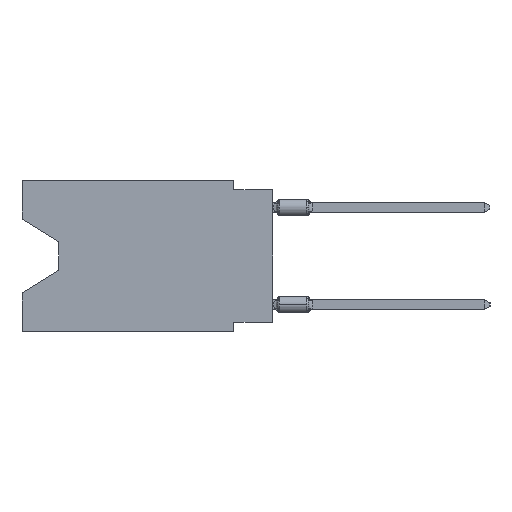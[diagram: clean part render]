
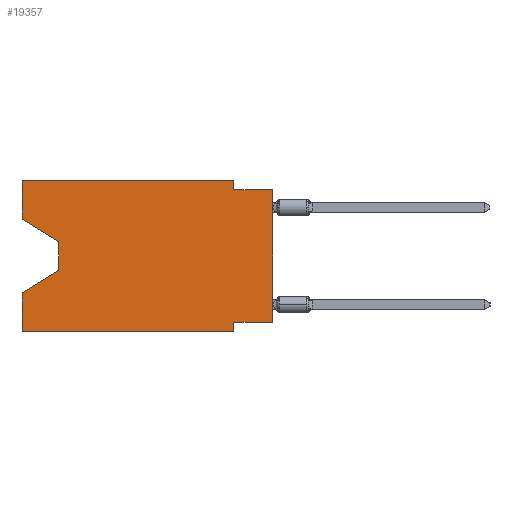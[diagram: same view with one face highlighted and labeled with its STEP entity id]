
A CAD part, left-side view. The second image highlights one B-rep face of the part: STEP entity #19357.
In plain terms, the highlighted planar face has unit normal (-1, 0, 0).
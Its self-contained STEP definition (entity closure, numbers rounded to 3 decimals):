
#1001 = CARTESIAN_POINT ( 'NONE',  ( 0., 0., -9.271 ) ) ;
#1278 = CARTESIAN_POINT ( 'NONE',  ( 0., 16.383, -9.906 ) ) ;
#1820 = CARTESIAN_POINT ( 'NONE',  ( 0., 16.383, 0. ) ) ;
#2032 = VERTEX_POINT ( 'NONE', #52408 ) ;
#2123 = EDGE_CURVE ( 'NONE', #40672, #59513, #11271, .T. ) ;
#3144 = CARTESIAN_POINT ( 'NONE',  ( 0., 2.54, -0.635 ) ) ;
#3154 = DIRECTION ( 'NONE',  ( 0., -0.855, -0.519 ) ) ;
#3254 = LINE ( 'NONE', #39486, #27759 ) ;
#4217 = DIRECTION ( 'NONE',  ( 0., 0., 1. ) ) ;
#4547 = VECTOR ( 'NONE', #3154, 1000. ) ;
#6039 = VECTOR ( 'NONE', #48702, 1000. ) ;
#7146 = LINE ( 'NONE', #20957, #4547 ) ;
#11271 = LINE ( 'NONE', #29998, #6039 ) ;
#11551 = CARTESIAN_POINT ( 'NONE',  ( 0., 13.97, -5.893 ) ) ;
#12085 = VECTOR ( 'NONE', #20526, 1000. ) ;
#12432 = VECTOR ( 'NONE', #40682, 1000. ) ;
#12573 = VECTOR ( 'NONE', #15448, 1000. ) ;
#12969 = EDGE_LOOP ( 'NONE', ( #15234, #33866, #51810, #21047, #34002, #48993, #49906, #43715, #22355, #38930, #28117, #49128 ) ) ;
#13271 = FACE_OUTER_BOUND ( 'NONE', #12969, .T. ) ;
#13844 = VECTOR ( 'NONE', #4217, 1000. ) ;
#14846 = CARTESIAN_POINT ( 'NONE',  ( 0., 2.54, -9.906 ) ) ;
#15234 = ORIENTED_EDGE ( 'NONE', *, *, #43062, .T. ) ;
#15448 = DIRECTION ( 'NONE',  ( 0., 0.855, -0.519 ) ) ;
#16613 = CARTESIAN_POINT ( 'NONE',  ( 0., 13.97, -4.013 ) ) ;
#17149 = CARTESIAN_POINT ( 'NONE',  ( 0., 0., -9.271 ) ) ;
#19357 = ADVANCED_FACE ( 'NONE', ( #13271 ), #56511, .F. ) ;
#19986 = DIRECTION ( 'NONE',  ( 0., -1., 0. ) ) ;
#20526 = DIRECTION ( 'NONE',  ( 0., -1., 0. ) ) ;
#20957 = CARTESIAN_POINT ( 'NONE',  ( 0., 16.383, -2.546 ) ) ;
#21047 = ORIENTED_EDGE ( 'NONE', *, *, #49150, .F. ) ;
#21268 = LINE ( 'NONE', #39997, #27341 ) ;
#22106 = DIRECTION ( 'NONE',  ( 0., 0., -1. ) ) ;
#22355 = ORIENTED_EDGE ( 'NONE', *, *, #46627, .F. ) ;
#23668 = CARTESIAN_POINT ( 'NONE',  ( 0., 16.383, 0. ) ) ;
#23907 = VECTOR ( 'NONE', #29219, 1000. ) ;
#25269 = DIRECTION ( 'NONE',  ( 0., -1., 0. ) ) ;
#27341 = VECTOR ( 'NONE', #25269, 1000. ) ;
#27759 = VECTOR ( 'NONE', #53586, 1000. ) ;
#28109 = CARTESIAN_POINT ( 'NONE',  ( 0., 16.383, -2.546 ) ) ;
#28117 = ORIENTED_EDGE ( 'NONE', *, *, #30103, .F. ) ;
#28427 = CARTESIAN_POINT ( 'NONE',  ( 0., 0., 0. ) ) ;
#29219 = DIRECTION ( 'NONE',  ( 0., 1., 0. ) ) ;
#29363 = CARTESIAN_POINT ( 'NONE',  ( 0., 2.54, -9.271 ) ) ;
#29998 = CARTESIAN_POINT ( 'NONE',  ( 0., 2.54, 0. ) ) ;
#30103 = EDGE_CURVE ( 'NONE', #42078, #40672, #43847, .T. ) ;
#30522 = VERTEX_POINT ( 'NONE', #29363 ) ;
#30609 = EDGE_CURVE ( 'NONE', #30522, #41639, #3254, .T. ) ;
#31034 = LINE ( 'NONE', #16613, #50163 ) ;
#31181 = LINE ( 'NONE', #55087, #12432 ) ;
#31206 = VERTEX_POINT ( 'NONE', #31725 ) ;
#31414 = AXIS2_PLACEMENT_3D ( 'NONE', #60206, #37490, #46390 ) ;
#31444 = EDGE_CURVE ( 'NONE', #39510, #30522, #43032, .T. ) ;
#31725 = CARTESIAN_POINT ( 'NONE',  ( 0., 0., -0.635 ) ) ;
#32756 = CARTESIAN_POINT ( 'NONE',  ( 0., 16.383, 0. ) ) ;
#33285 = EDGE_CURVE ( 'NONE', #39510, #31206, #42555, .T. ) ;
#33498 = LINE ( 'NONE', #1278, #36213 ) ;
#33535 = CARTESIAN_POINT ( 'NONE',  ( 0., 13.97, -4.013 ) ) ;
#33866 = ORIENTED_EDGE ( 'NONE', *, *, #49960, .T. ) ;
#33870 = LINE ( 'NONE', #52863, #12573 ) ;
#34002 = ORIENTED_EDGE ( 'NONE', *, *, #37813, .T. ) ;
#34744 = EDGE_CURVE ( 'NONE', #55084, #42078, #31181, .T. ) ;
#35126 = VERTEX_POINT ( 'NONE', #38496 ) ;
#36213 = VECTOR ( 'NONE', #19986, 1000. ) ;
#37490 = DIRECTION ( 'NONE',  ( 1., 0., 0. ) ) ;
#37813 = EDGE_CURVE ( 'NONE', #2032, #41639, #33498, .T. ) ;
#38496 = CARTESIAN_POINT ( 'NONE',  ( 0., 16.383, -7.36 ) ) ;
#38930 = ORIENTED_EDGE ( 'NONE', *, *, #2123, .F. ) ;
#39486 = CARTESIAN_POINT ( 'NONE',  ( 0., 2.54, -9.906 ) ) ;
#39510 = VERTEX_POINT ( 'NONE', #17149 ) ;
#39997 = CARTESIAN_POINT ( 'NONE',  ( 0., 0., -0.635 ) ) ;
#40672 = VERTEX_POINT ( 'NONE', #50676 ) ;
#40682 = DIRECTION ( 'NONE',  ( 0., 0., 1. ) ) ;
#41639 = VERTEX_POINT ( 'NONE', #14846 ) ;
#42078 = VERTEX_POINT ( 'NONE', #23668 ) ;
#42555 = LINE ( 'NONE', #28427, #43659 ) ;
#43032 = LINE ( 'NONE', #1001, #23907 ) ;
#43062 = EDGE_CURVE ( 'NONE', #55084, #60505, #7146, .T. ) ;
#43659 = VECTOR ( 'NONE', #56054, 1000. ) ;
#43715 = ORIENTED_EDGE ( 'NONE', *, *, #33285, .T. ) ;
#43847 = LINE ( 'NONE', #1820, #12085 ) ;
#46390 = DIRECTION ( 'NONE',  ( 0., 0., -1. ) ) ;
#46627 = EDGE_CURVE ( 'NONE', #59513, #31206, #21268, .T. ) ;
#48702 = DIRECTION ( 'NONE',  ( 0., 0., -1. ) ) ;
#48993 = ORIENTED_EDGE ( 'NONE', *, *, #30609, .F. ) ;
#49128 = ORIENTED_EDGE ( 'NONE', *, *, #34744, .F. ) ;
#49150 = EDGE_CURVE ( 'NONE', #2032, #35126, #60362, .T. ) ;
#49906 = ORIENTED_EDGE ( 'NONE', *, *, #31444, .F. ) ;
#49960 = EDGE_CURVE ( 'NONE', #60505, #51993, #31034, .T. ) ;
#50163 = VECTOR ( 'NONE', #22106, 1000. ) ;
#50676 = CARTESIAN_POINT ( 'NONE',  ( 0., 2.54, 0. ) ) ;
#51810 = ORIENTED_EDGE ( 'NONE', *, *, #53923, .T. ) ;
#51993 = VERTEX_POINT ( 'NONE', #11551 ) ;
#52408 = CARTESIAN_POINT ( 'NONE',  ( 0., 16.383, -9.906 ) ) ;
#52863 = CARTESIAN_POINT ( 'NONE',  ( 0., 13.97, -5.893 ) ) ;
#53586 = DIRECTION ( 'NONE',  ( 0., 0., -1. ) ) ;
#53923 = EDGE_CURVE ( 'NONE', #51993, #35126, #33870, .T. ) ;
#55084 = VERTEX_POINT ( 'NONE', #28109 ) ;
#55087 = CARTESIAN_POINT ( 'NONE',  ( 0., 16.383, 0. ) ) ;
#56054 = DIRECTION ( 'NONE',  ( 0., 0., 1. ) ) ;
#56511 = PLANE ( 'NONE',  #31414 ) ;
#59513 = VERTEX_POINT ( 'NONE', #3144 ) ;
#60206 = CARTESIAN_POINT ( 'NONE',  ( 0., 16.383, 0. ) ) ;
#60362 = LINE ( 'NONE', #32756, #13844 ) ;
#60505 = VERTEX_POINT ( 'NONE', #33535 ) ;
